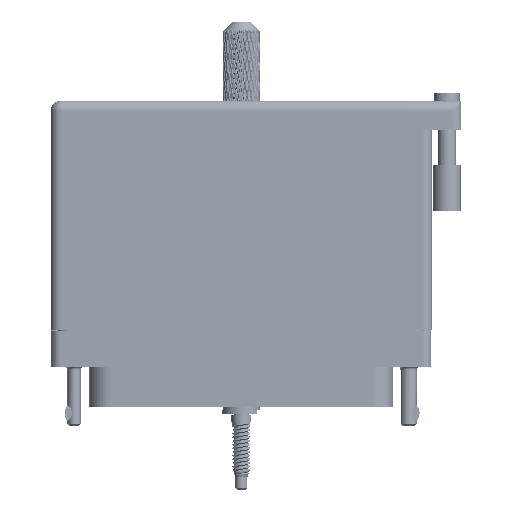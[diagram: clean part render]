
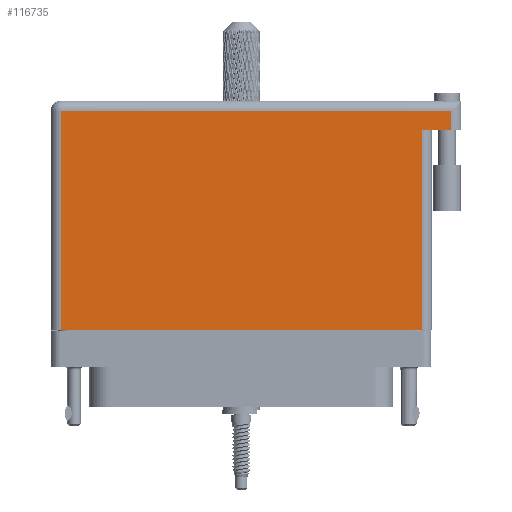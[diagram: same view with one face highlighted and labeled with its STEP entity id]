
A CAD part, front view. The second image highlights one B-rep face of the part: STEP entity #116735.
In plain terms, the highlighted face is planar.
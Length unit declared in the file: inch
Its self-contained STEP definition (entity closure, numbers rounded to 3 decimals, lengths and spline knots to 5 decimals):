
#1165 = EDGE_CURVE ( 'NONE', #5718, #36947, #14900, .T. ) ;
#5610 = EDGE_CURVE ( 'NONE', #77950, #110046, #34068, .T. ) ;
#5718 = VERTEX_POINT ( 'NONE', #78415 ) ;
#10466 = VERTEX_POINT ( 'NONE', #95506 ) ;
#11625 = VECTOR ( 'NONE', #57106, 39.37008 ) ;
#14900 = LINE ( 'NONE', #39115, #63656 ) ;
#15222 = EDGE_CURVE ( 'NONE', #64291, #77950, #38777, .T. ) ;
#17057 = CARTESIAN_POINT ( 'NONE',  ( -1.3, 1.396, 0.4495 ) ) ;
#18634 = ORIENTED_EDGE ( 'NONE', *, *, #5610, .T. ) ;
#24510 = CARTESIAN_POINT ( 'NONE',  ( 1.5, 1.269, 0.4495 ) ) ;
#24532 = EDGE_CURVE ( 'NONE', #64291, #10466, #36433, .T. ) ;
#24577 = FACE_OUTER_BOUND ( 'NONE', #73371, .T. ) ;
#24899 = CARTESIAN_POINT ( 'NONE',  ( -1.23, -0.1, 0.4495 ) ) ;
#26518 = VECTOR ( 'NONE', #77916, 39.37008 ) ;
#33847 = CARTESIAN_POINT ( 'NONE',  ( -1.23, 1.396, 0.4495 ) ) ;
#34068 = LINE ( 'NONE', #17057, #37090 ) ;
#36433 = LINE ( 'NONE', #24510, #37893 ) ;
#36764 = ORIENTED_EDGE ( 'NONE', *, *, #1165, .T. ) ;
#36947 = VERTEX_POINT ( 'NONE', #75938 ) ;
#37090 = VECTOR ( 'NONE', #115306, 39.37008 ) ;
#37893 = VECTOR ( 'NONE', #54308, 39.37008 ) ;
#38777 = LINE ( 'NONE', #68104, #26518 ) ;
#39115 = CARTESIAN_POINT ( 'NONE',  ( -1.3, -0.1, 0.4495 ) ) ;
#42024 = EDGE_CURVE ( 'NONE', #110046, #5718, #98813, .T. ) ;
#43158 = EDGE_CURVE ( 'NONE', #36947, #10466, #63404, .T. ) ;
#44517 = DIRECTION ( 'NONE',  ( 0., -1., 0. ) ) ;
#51687 = DIRECTION ( 'NONE',  ( -1., 0., 0. ) ) ;
#54308 = DIRECTION ( 'NONE',  ( -1., 0., 0. ) ) ;
#54861 = ORIENTED_EDGE ( 'NONE', *, *, #24532, .F. ) ;
#57106 = DIRECTION ( 'NONE',  ( 0., 1., 0. ) ) ;
#57807 = DIRECTION ( 'NONE',  ( 1., 0., 0. ) ) ;
#63404 = LINE ( 'NONE', #96076, #11625 ) ;
#63656 = VECTOR ( 'NONE', #57807, 39.37008 ) ;
#64291 = VERTEX_POINT ( 'NONE', #68641 ) ;
#68104 = CARTESIAN_POINT ( 'NONE',  ( 1.43, 1.466, 0.4495 ) ) ;
#68641 = CARTESIAN_POINT ( 'NONE',  ( 1.43, 1.269, 0.4495 ) ) ;
#69597 = CARTESIAN_POINT ( 'NONE',  ( -1.3, 1.466, 0.4495 ) ) ;
#73371 = EDGE_LOOP ( 'NONE', ( #36764, #108548, #54861, #74692, #18634, #109536 ) ) ;
#73515 = AXIS2_PLACEMENT_3D ( 'NONE', #69597, #109392, #51687 ) ;
#74692 = ORIENTED_EDGE ( 'NONE', *, *, #15222, .T. ) ;
#75938 = CARTESIAN_POINT ( 'NONE',  ( 1.23, -0.1, 0.4495 ) ) ;
#77916 = DIRECTION ( 'NONE',  ( 0., 1., 0. ) ) ;
#77950 = VERTEX_POINT ( 'NONE', #88036 ) ;
#78415 = CARTESIAN_POINT ( 'NONE',  ( -1.23, -0.1, 0.4495 ) ) ;
#83408 = VECTOR ( 'NONE', #44517, 39.37008 ) ;
#85463 = PLANE ( 'NONE',  #73515 ) ;
#88036 = CARTESIAN_POINT ( 'NONE',  ( 1.43, 1.396, 0.4495 ) ) ;
#95506 = CARTESIAN_POINT ( 'NONE',  ( 1.23, 1.269, 0.4495 ) ) ;
#96076 = CARTESIAN_POINT ( 'NONE',  ( 1.23, 1.269, 0.4495 ) ) ;
#98813 = LINE ( 'NONE', #24899, #83408 ) ;
#108548 = ORIENTED_EDGE ( 'NONE', *, *, #43158, .T. ) ;
#109392 = DIRECTION ( 'NONE',  ( 0., 0., -1. ) ) ;
#109536 = ORIENTED_EDGE ( 'NONE', *, *, #42024, .T. ) ;
#110046 = VERTEX_POINT ( 'NONE', #33847 ) ;
#115306 = DIRECTION ( 'NONE',  ( -1., 0., 0. ) ) ;
#116735 = ADVANCED_FACE ( 'NONE', ( #24577 ), #85463, .F. ) ;
